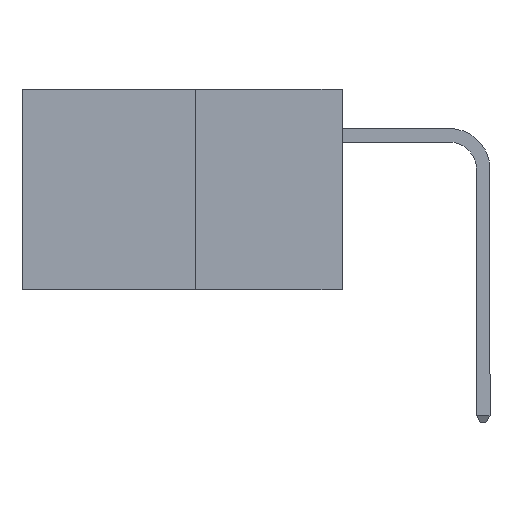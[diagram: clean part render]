
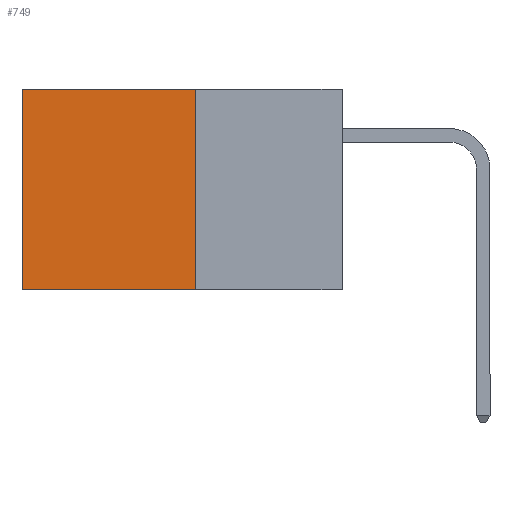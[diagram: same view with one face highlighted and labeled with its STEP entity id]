
A CAD part, left-side view. The second image highlights one B-rep face of the part: STEP entity #749.
In plain terms, the highlighted planar face has unit normal (-1, 0, 0).
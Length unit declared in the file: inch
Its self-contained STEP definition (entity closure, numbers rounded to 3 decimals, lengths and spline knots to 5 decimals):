
#600 = AXIS2_PLACEMENT_3D ( 'NONE', #5565, #1307, #6751 ) ;
#749 = ADVANCED_FACE ( 'NONE', ( #1922 ), #2982, .F. ) ;
#892 = EDGE_LOOP ( 'NONE', ( #1642, #6729, #2026, #2229 ) ) ;
#949 = EDGE_CURVE ( 'NONE', #4491, #4718, #4043, .T. ) ;
#1307 = DIRECTION ( 'NONE',  ( 1., 0., 0. ) ) ;
#1526 = CARTESIAN_POINT ( 'NONE',  ( 0.277, 0.59, -0.37 ) ) ;
#1642 = ORIENTED_EDGE ( 'NONE', *, *, #4136, .T. ) ;
#1666 = LINE ( 'NONE', #1526, #7771 ) ;
#1922 = FACE_OUTER_BOUND ( 'NONE', #892, .T. ) ;
#2026 = ORIENTED_EDGE ( 'NONE', *, *, #4428, .F. ) ;
#2229 = ORIENTED_EDGE ( 'NONE', *, *, #949, .T. ) ;
#2497 = DIRECTION ( 'NONE',  ( 0., 0., -1. ) ) ;
#2542 = VECTOR ( 'NONE', #7427, 39.37008 ) ;
#2638 = CARTESIAN_POINT ( 'NONE',  ( 0.277, 0.27, -0.37 ) ) ;
#2982 = PLANE ( 'NONE',  #600 ) ;
#3108 = CARTESIAN_POINT ( 'NONE',  ( 0.277, 0.27, -0.37 ) ) ;
#4043 = LINE ( 'NONE', #6825, #5652 ) ;
#4136 = EDGE_CURVE ( 'NONE', #4718, #5356, #1666, .T. ) ;
#4428 = EDGE_CURVE ( 'NONE', #4491, #4818, #6193, .T. ) ;
#4491 = VERTEX_POINT ( 'NONE', #5981 ) ;
#4525 = LINE ( 'NONE', #7514, #2542 ) ;
#4718 = VERTEX_POINT ( 'NONE', #6466 ) ;
#4818 = VERTEX_POINT ( 'NONE', #2638 ) ;
#4984 = DIRECTION ( 'NONE',  ( 0., 0., -1. ) ) ;
#4996 = CARTESIAN_POINT ( 'NONE',  ( 0.277, 0.59, -0.37 ) ) ;
#5356 = VERTEX_POINT ( 'NONE', #4996 ) ;
#5565 = CARTESIAN_POINT ( 'NONE',  ( 0.277, 0.27, -0.37 ) ) ;
#5652 = VECTOR ( 'NONE', #6329, 39.37008 ) ;
#5981 = CARTESIAN_POINT ( 'NONE',  ( 0.277, 0.27, 0. ) ) ;
#6193 = LINE ( 'NONE', #3108, #7368 ) ;
#6329 = DIRECTION ( 'NONE',  ( 0., 1., 0. ) ) ;
#6466 = CARTESIAN_POINT ( 'NONE',  ( 0.277, 0.59, 0. ) ) ;
#6545 = EDGE_CURVE ( 'NONE', #4818, #5356, #4525, .T. ) ;
#6729 = ORIENTED_EDGE ( 'NONE', *, *, #6545, .F. ) ;
#6751 = DIRECTION ( 'NONE',  ( 0., 0., -1. ) ) ;
#6825 = CARTESIAN_POINT ( 'NONE',  ( 0.277, 0.27, 0. ) ) ;
#7368 = VECTOR ( 'NONE', #2497, 39.37008 ) ;
#7427 = DIRECTION ( 'NONE',  ( 0., 1., 0. ) ) ;
#7514 = CARTESIAN_POINT ( 'NONE',  ( 0.277, 0.27, -0.37 ) ) ;
#7771 = VECTOR ( 'NONE', #4984, 39.37008 ) ;
